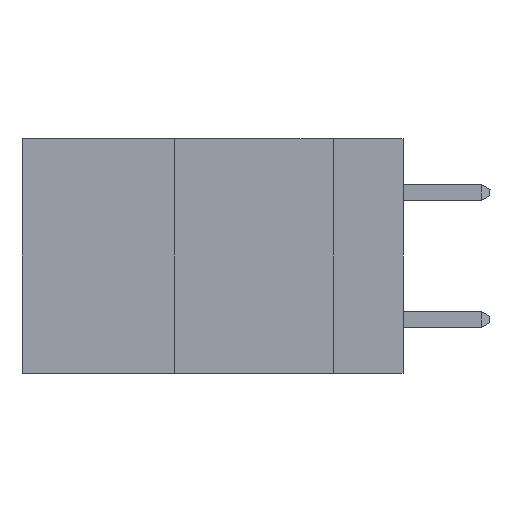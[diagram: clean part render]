
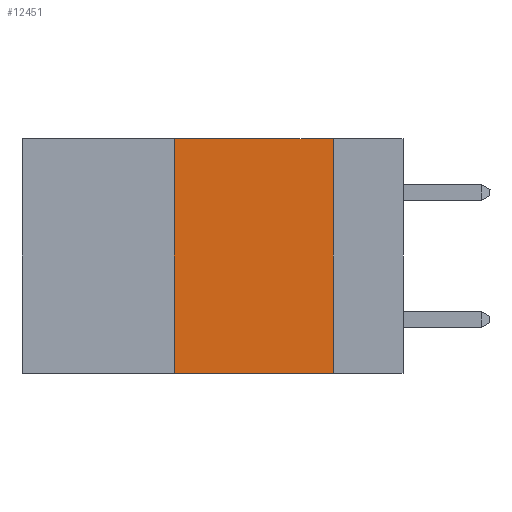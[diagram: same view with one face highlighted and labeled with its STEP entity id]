
A CAD part, left-side view. The second image highlights one B-rep face of the part: STEP entity #12451.
In plain terms, the highlighted planar face has unit normal (-1, 0, 0).
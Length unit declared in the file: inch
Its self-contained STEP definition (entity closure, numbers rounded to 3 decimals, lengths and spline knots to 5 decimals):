
#762 = ORIENTED_EDGE ( 'NONE', *, *, #15848, .F. ) ;
#2206 = VECTOR ( 'NONE', #10542, 39.37008 ) ;
#2207 = CARTESIAN_POINT ( 'NONE',  ( 0., 0.36, 0. ) ) ;
#2233 = CARTESIAN_POINT ( 'NONE',  ( 0., 0.36, -0.37 ) ) ;
#2766 = ORIENTED_EDGE ( 'NONE', *, *, #12313, .F. ) ;
#3553 = LINE ( 'NONE', #21644, #2206 ) ;
#4275 = FACE_OUTER_BOUND ( 'NONE', #13586, .T. ) ;
#4762 = VERTEX_POINT ( 'NONE', #16732 ) ;
#5041 = EDGE_CURVE ( 'NONE', #4762, #26127, #3553, .T. ) ;
#5129 = EDGE_CURVE ( 'NONE', #12799, #25453, #22833, .T. ) ;
#6629 = CARTESIAN_POINT ( 'NONE',  ( 0., 0.11, 0. ) ) ;
#6795 = VECTOR ( 'NONE', #15148, 39.37008 ) ;
#7331 = LINE ( 'NONE', #2207, #24289 ) ;
#7369 = DIRECTION ( 'NONE',  ( 0., 0., -1. ) ) ;
#10477 = LINE ( 'NONE', #6629, #6795 ) ;
#10519 = AXIS2_PLACEMENT_3D ( 'NONE', #13513, #11432, #7369 ) ;
#10542 = DIRECTION ( 'NONE',  ( 0., -1., 0. ) ) ;
#11348 = PLANE ( 'NONE',  #10519 ) ;
#11432 = DIRECTION ( 'NONE',  ( 1., 0., 0. ) ) ;
#11960 = VECTOR ( 'NONE', #26228, 39.37008 ) ;
#12313 = EDGE_CURVE ( 'NONE', #12799, #4762, #7331, .T. ) ;
#12451 = ADVANCED_FACE ( 'NONE', ( #4275 ), #11348, .F. ) ;
#12799 = VERTEX_POINT ( 'NONE', #2233 ) ;
#13513 = CARTESIAN_POINT ( 'NONE',  ( 0., 0.6, 0. ) ) ;
#13586 = EDGE_LOOP ( 'NONE', ( #762, #21167, #2766, #17740 ) ) ;
#15148 = DIRECTION ( 'NONE',  ( 0., 0., -1. ) ) ;
#15848 = EDGE_CURVE ( 'NONE', #26127, #25453, #10477, .T. ) ;
#16732 = CARTESIAN_POINT ( 'NONE',  ( 0., 0.36, 0. ) ) ;
#17706 = CARTESIAN_POINT ( 'NONE',  ( 0., 0.6, -0.37 ) ) ;
#17740 = ORIENTED_EDGE ( 'NONE', *, *, #5129, .T. ) ;
#21167 = ORIENTED_EDGE ( 'NONE', *, *, #5041, .F. ) ;
#21644 = CARTESIAN_POINT ( 'NONE',  ( 0., 0.6, 0. ) ) ;
#22833 = LINE ( 'NONE', #17706, #11960 ) ;
#23857 = DIRECTION ( 'NONE',  ( 0., 0., 1. ) ) ;
#24038 = CARTESIAN_POINT ( 'NONE',  ( 0., 0.11, 0. ) ) ;
#24289 = VECTOR ( 'NONE', #23857, 39.37008 ) ;
#25149 = CARTESIAN_POINT ( 'NONE',  ( 0., 0.11, -0.37 ) ) ;
#25453 = VERTEX_POINT ( 'NONE', #25149 ) ;
#26127 = VERTEX_POINT ( 'NONE', #24038 ) ;
#26228 = DIRECTION ( 'NONE',  ( 0., -1., 0. ) ) ;
